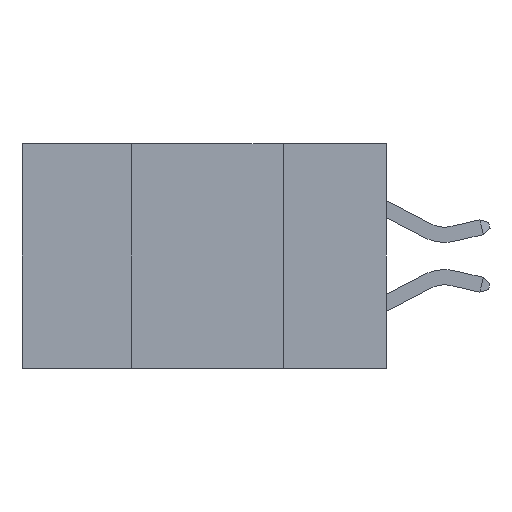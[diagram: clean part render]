
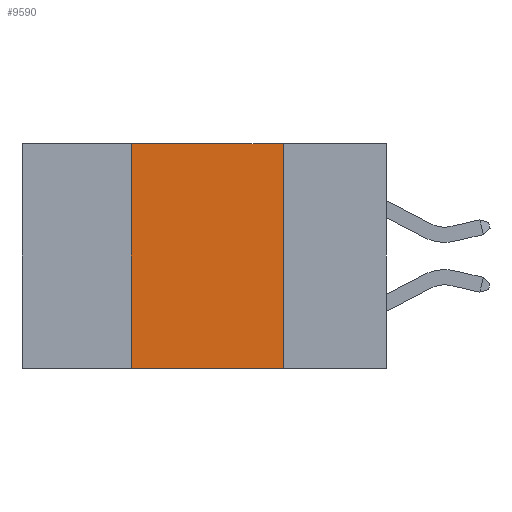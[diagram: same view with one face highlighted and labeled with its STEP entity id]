
A CAD part, left-side view. The second image highlights one B-rep face of the part: STEP entity #9590.
In plain terms, the highlighted planar face has unit normal (-1, 0, 0).
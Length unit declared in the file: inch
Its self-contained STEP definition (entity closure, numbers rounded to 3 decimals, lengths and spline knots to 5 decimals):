
#190 = VECTOR ( 'NONE', #10751, 39.37008 ) ;
#347 = CARTESIAN_POINT ( 'NONE',  ( 0., 0.6, 0. ) ) ;
#1309 = DIRECTION ( 'NONE',  ( 1., 0., 0. ) ) ;
#1382 = EDGE_CURVE ( 'NONE', #6688, #7526, #7924, .T. ) ;
#1536 = CARTESIAN_POINT ( 'NONE',  ( 0., 0.17, -0.37 ) ) ;
#1681 = CARTESIAN_POINT ( 'NONE',  ( 0., 0.42, -0.37 ) ) ;
#1716 = CARTESIAN_POINT ( 'NONE',  ( 0., 0.42, 0. ) ) ;
#1786 = EDGE_LOOP ( 'NONE', ( #8986, #6762, #11685, #4524 ) ) ;
#2725 = EDGE_CURVE ( 'NONE', #6688, #3921, #2781, .T. ) ;
#2781 = LINE ( 'NONE', #5873, #7587 ) ;
#2818 = DIRECTION ( 'NONE',  ( 0., -1., 0. ) ) ;
#3358 = DIRECTION ( 'NONE',  ( 0., 0., 1. ) ) ;
#3485 = AXIS2_PLACEMENT_3D ( 'NONE', #347, #1309, #8098 ) ;
#3921 = VERTEX_POINT ( 'NONE', #1716 ) ;
#4132 = EDGE_CURVE ( 'NONE', #8698, #7526, #10600, .T. ) ;
#4524 = ORIENTED_EDGE ( 'NONE', *, *, #1382, .T. ) ;
#5036 = FACE_OUTER_BOUND ( 'NONE', #1786, .T. ) ;
#5312 = CARTESIAN_POINT ( 'NONE',  ( 0., 0.6, -0.37 ) ) ;
#5873 = CARTESIAN_POINT ( 'NONE',  ( 0., 0.42, 0. ) ) ;
#6178 = PLANE ( 'NONE',  #3485 ) ;
#6688 = VERTEX_POINT ( 'NONE', #1681 ) ;
#6762 = ORIENTED_EDGE ( 'NONE', *, *, #8206, .F. ) ;
#6813 = LINE ( 'NONE', #7596, #11738 ) ;
#7353 = CARTESIAN_POINT ( 'NONE',  ( 0., 0.17, 0. ) ) ;
#7526 = VERTEX_POINT ( 'NONE', #1536 ) ;
#7587 = VECTOR ( 'NONE', #3358, 39.37008 ) ;
#7596 = CARTESIAN_POINT ( 'NONE',  ( 0., 0.6, 0. ) ) ;
#7924 = LINE ( 'NONE', #5312, #190 ) ;
#8098 = DIRECTION ( 'NONE',  ( 0., 0., -1. ) ) ;
#8156 = VECTOR ( 'NONE', #12230, 39.37008 ) ;
#8206 = EDGE_CURVE ( 'NONE', #3921, #8698, #6813, .T. ) ;
#8275 = CARTESIAN_POINT ( 'NONE',  ( 0., 0.17, 0. ) ) ;
#8698 = VERTEX_POINT ( 'NONE', #8275 ) ;
#8986 = ORIENTED_EDGE ( 'NONE', *, *, #4132, .F. ) ;
#9590 = ADVANCED_FACE ( 'NONE', ( #5036 ), #6178, .F. ) ;
#10600 = LINE ( 'NONE', #7353, #8156 ) ;
#10751 = DIRECTION ( 'NONE',  ( 0., -1., 0. ) ) ;
#11685 = ORIENTED_EDGE ( 'NONE', *, *, #2725, .F. ) ;
#11738 = VECTOR ( 'NONE', #2818, 39.37008 ) ;
#12230 = DIRECTION ( 'NONE',  ( 0., 0., -1. ) ) ;
